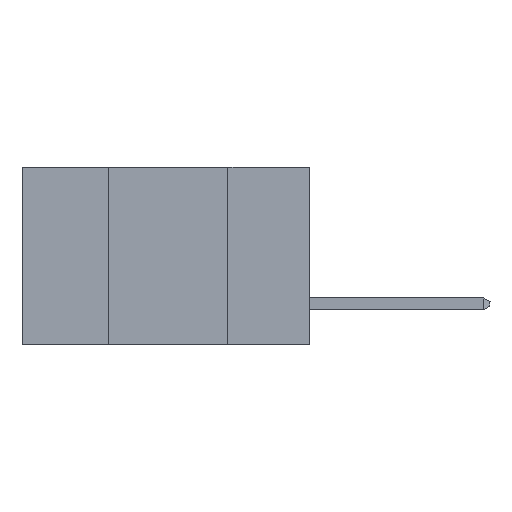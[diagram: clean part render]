
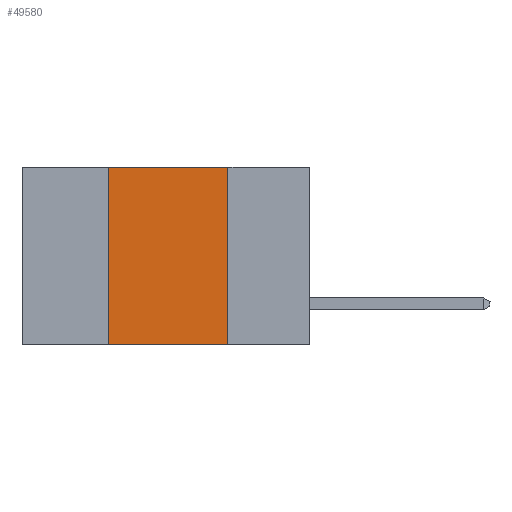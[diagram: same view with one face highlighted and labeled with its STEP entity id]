
A CAD part, left-side view. The second image highlights one B-rep face of the part: STEP entity #49580.
In plain terms, the highlighted planar face has unit normal (-1, 0, 0).
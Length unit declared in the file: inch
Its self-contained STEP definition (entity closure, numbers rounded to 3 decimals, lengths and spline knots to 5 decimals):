
#1294 = ORIENTED_EDGE ( 'NONE', *, *, #45416, .F. ) ;
#1359 = VECTOR ( 'NONE', #34111, 39.37008 ) ;
#1996 = ORIENTED_EDGE ( 'NONE', *, *, #44411, .F. ) ;
#3781 = VECTOR ( 'NONE', #14053, 39.37008 ) ;
#5167 = LINE ( 'NONE', #44688, #44592 ) ;
#7648 = FACE_OUTER_BOUND ( 'NONE', #12730, .T. ) ;
#8876 = ORIENTED_EDGE ( 'NONE', *, *, #32252, .T. ) ;
#12484 = EDGE_CURVE ( 'NONE', #37028, #24607, #5167, .T. ) ;
#12730 = EDGE_LOOP ( 'NONE', ( #1996, #1294, #14372, #8876 ) ) ;
#14053 = DIRECTION ( 'NONE',  ( 0., -1., 0. ) ) ;
#14372 = ORIENTED_EDGE ( 'NONE', *, *, #12484, .F. ) ;
#15131 = VERTEX_POINT ( 'NONE', #33472 ) ;
#15367 = DIRECTION ( 'NONE',  ( 0., 0., -1. ) ) ;
#18458 = LINE ( 'NONE', #22570, #1359 ) ;
#18733 = AXIS2_PLACEMENT_3D ( 'NONE', #50253, #50508, #15367 ) ;
#21514 = CARTESIAN_POINT ( 'NONE',  ( 0., 0.42, 0. ) ) ;
#22570 = CARTESIAN_POINT ( 'NONE',  ( 0., 0.6, -0.37 ) ) ;
#23525 = DIRECTION ( 'NONE',  ( 0., 0., -1. ) ) ;
#24487 = VERTEX_POINT ( 'NONE', #43830 ) ;
#24536 = CARTESIAN_POINT ( 'NONE',  ( 0., 0.17, 0. ) ) ;
#24607 = VERTEX_POINT ( 'NONE', #21514 ) ;
#29781 = CARTESIAN_POINT ( 'NONE',  ( 0., 0.42, -0.37 ) ) ;
#32252 = EDGE_CURVE ( 'NONE', #37028, #15131, #18458, .T. ) ;
#32610 = LINE ( 'NONE', #41754, #3781 ) ;
#33472 = CARTESIAN_POINT ( 'NONE',  ( 0., 0.17, -0.37 ) ) ;
#34111 = DIRECTION ( 'NONE',  ( 0., -1., 0. ) ) ;
#34608 = PLANE ( 'NONE',  #18733 ) ;
#36479 = DIRECTION ( 'NONE',  ( 0., 0., 1. ) ) ;
#37028 = VERTEX_POINT ( 'NONE', #29781 ) ;
#39758 = VECTOR ( 'NONE', #23525, 39.37008 ) ;
#41754 = CARTESIAN_POINT ( 'NONE',  ( 0., 0.6, 0. ) ) ;
#43830 = CARTESIAN_POINT ( 'NONE',  ( 0., 0.17, 0. ) ) ;
#44411 = EDGE_CURVE ( 'NONE', #24487, #15131, #47858, .T. ) ;
#44592 = VECTOR ( 'NONE', #36479, 39.37008 ) ;
#44688 = CARTESIAN_POINT ( 'NONE',  ( 0., 0.42, 0. ) ) ;
#45416 = EDGE_CURVE ( 'NONE', #24607, #24487, #32610, .T. ) ;
#47858 = LINE ( 'NONE', #24536, #39758 ) ;
#49580 = ADVANCED_FACE ( 'NONE', ( #7648 ), #34608, .F. ) ;
#50253 = CARTESIAN_POINT ( 'NONE',  ( 0., 0.6, 0. ) ) ;
#50508 = DIRECTION ( 'NONE',  ( 1., 0., 0. ) ) ;
